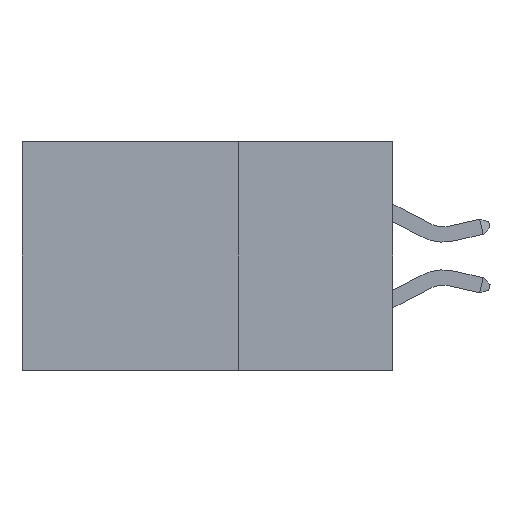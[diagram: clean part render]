
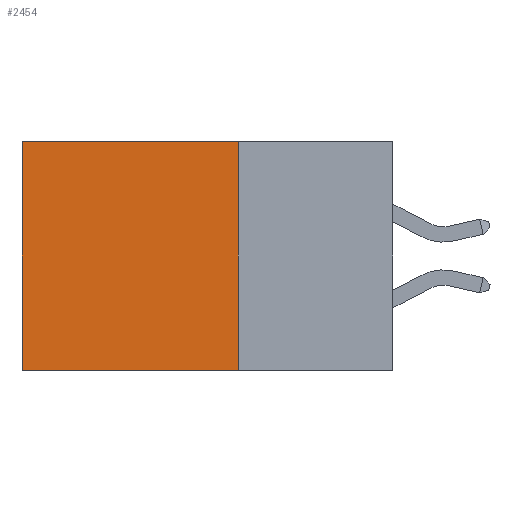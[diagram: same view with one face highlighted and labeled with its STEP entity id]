
A CAD part, left-side view. The second image highlights one B-rep face of the part: STEP entity #2454.
In plain terms, the highlighted planar face has unit normal (-1, 0, 0).
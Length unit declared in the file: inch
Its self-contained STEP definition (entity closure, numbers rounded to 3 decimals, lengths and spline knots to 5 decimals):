
#1110 = ORIENTED_EDGE ( 'NONE', *, *, #13663, .T. ) ;
#1312 = PLANE ( 'NONE',  #11159 ) ;
#1429 = CARTESIAN_POINT ( 'NONE',  ( 0.2875, 0.25, 0. ) ) ;
#1942 = LINE ( 'NONE', #10913, #25838 ) ;
#2454 = ADVANCED_FACE ( 'NONE', ( #30770 ), #1312, .F. ) ;
#4842 = LINE ( 'NONE', #6155, #30729 ) ;
#4945 = DIRECTION ( 'NONE',  ( 0., 1., 0. ) ) ;
#5954 = CARTESIAN_POINT ( 'NONE',  ( 0.2875, 0.6, 0. ) ) ;
#6155 = CARTESIAN_POINT ( 'NONE',  ( 0.2875, 0.6, 0. ) ) ;
#7924 = EDGE_LOOP ( 'NONE', ( #20515, #18955, #9752, #1110 ) ) ;
#8405 = EDGE_CURVE ( 'NONE', #13526, #16104, #11072, .T. ) ;
#9752 = ORIENTED_EDGE ( 'NONE', *, *, #17904, .F. ) ;
#10683 = CARTESIAN_POINT ( 'NONE',  ( 0.2875, 0.25, -0.37 ) ) ;
#10913 = CARTESIAN_POINT ( 'NONE',  ( 0.2875, 0.25, 0. ) ) ;
#11072 = LINE ( 'NONE', #19905, #30372 ) ;
#11092 = CARTESIAN_POINT ( 'NONE',  ( 0.2875, 0.25, 0. ) ) ;
#11159 = AXIS2_PLACEMENT_3D ( 'NONE', #1429, #11356, #18913 ) ;
#11356 = DIRECTION ( 'NONE',  ( 1., 0., 0. ) ) ;
#12370 = VERTEX_POINT ( 'NONE', #5954 ) ;
#13526 = VERTEX_POINT ( 'NONE', #10683 ) ;
#13663 = EDGE_CURVE ( 'NONE', #14442, #12370, #22580, .T. ) ;
#14442 = VERTEX_POINT ( 'NONE', #19378 ) ;
#15949 = EDGE_CURVE ( 'NONE', #12370, #16104, #4842, .T. ) ;
#16104 = VERTEX_POINT ( 'NONE', #26989 ) ;
#17904 = EDGE_CURVE ( 'NONE', #14442, #13526, #1942, .T. ) ;
#18598 = VECTOR ( 'NONE', #31247, 39.37008 ) ;
#18728 = DIRECTION ( 'NONE',  ( 0., 0., -1. ) ) ;
#18913 = DIRECTION ( 'NONE',  ( 0., 0., -1. ) ) ;
#18955 = ORIENTED_EDGE ( 'NONE', *, *, #8405, .F. ) ;
#19378 = CARTESIAN_POINT ( 'NONE',  ( 0.2875, 0.25, 0. ) ) ;
#19905 = CARTESIAN_POINT ( 'NONE',  ( 0.2875, 0.25, -0.37 ) ) ;
#20515 = ORIENTED_EDGE ( 'NONE', *, *, #15949, .T. ) ;
#22580 = LINE ( 'NONE', #11092, #18598 ) ;
#25838 = VECTOR ( 'NONE', #31166, 39.37008 ) ;
#26989 = CARTESIAN_POINT ( 'NONE',  ( 0.2875, 0.6, -0.37 ) ) ;
#30372 = VECTOR ( 'NONE', #4945, 39.37008 ) ;
#30729 = VECTOR ( 'NONE', #18728, 39.37008 ) ;
#30770 = FACE_OUTER_BOUND ( 'NONE', #7924, .T. ) ;
#31166 = DIRECTION ( 'NONE',  ( 0., 0., -1. ) ) ;
#31247 = DIRECTION ( 'NONE',  ( 0., 1., 0. ) ) ;
